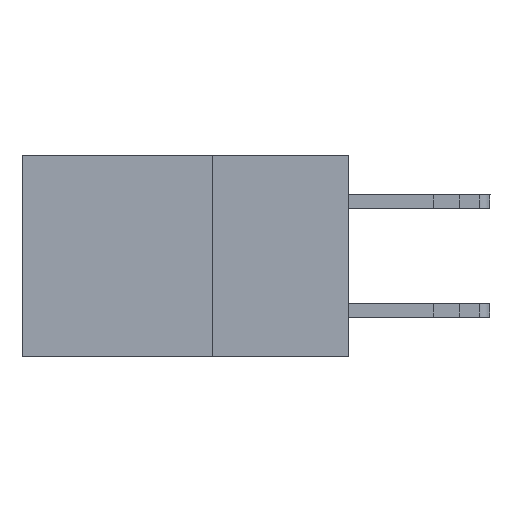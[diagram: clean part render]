
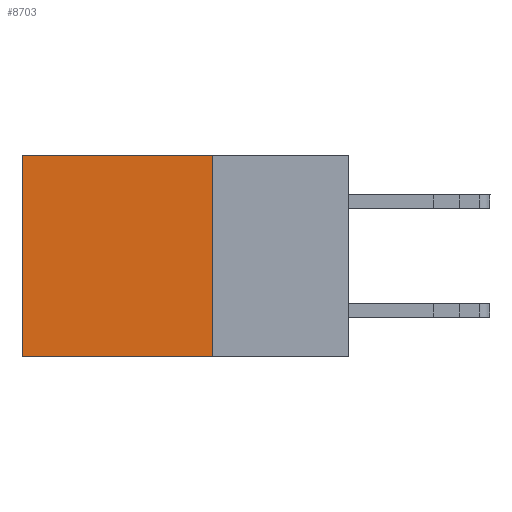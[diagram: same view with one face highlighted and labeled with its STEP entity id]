
A CAD part, left-side view. The second image highlights one B-rep face of the part: STEP entity #8703.
In plain terms, the highlighted planar face has unit normal (-1, 0, 0).
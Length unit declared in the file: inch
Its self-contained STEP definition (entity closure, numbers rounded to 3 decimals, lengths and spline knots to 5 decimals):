
#602 = CARTESIAN_POINT ( 'NONE',  ( 0.298, 0.6, 0. ) ) ;
#836 = EDGE_CURVE ( 'NONE', #10375, #9872, #7836, .T. ) ;
#1963 = DIRECTION ( 'NONE',  ( 0., 0., -1. ) ) ;
#2125 = LINE ( 'NONE', #4439, #6090 ) ;
#2302 = ORIENTED_EDGE ( 'NONE', *, *, #11563, .T. ) ;
#2629 = AXIS2_PLACEMENT_3D ( 'NONE', #14100, #3195, #12896 ) ;
#3061 = LINE ( 'NONE', #7759, #5135 ) ;
#3195 = DIRECTION ( 'NONE',  ( 1., 0., 0. ) ) ;
#3218 = DIRECTION ( 'NONE',  ( 0., 1., 0. ) ) ;
#3538 = CARTESIAN_POINT ( 'NONE',  ( 0.298, 0.25, 0. ) ) ;
#3546 = VECTOR ( 'NONE', #1963, 39.37008 ) ;
#3969 = EDGE_CURVE ( 'NONE', #10375, #10955, #15333, .T. ) ;
#3998 = EDGE_CURVE ( 'NONE', #10955, #11272, #2125, .T. ) ;
#4439 = CARTESIAN_POINT ( 'NONE',  ( 0.298, 0.25, -0.37 ) ) ;
#4466 = ORIENTED_EDGE ( 'NONE', *, *, #3969, .F. ) ;
#5135 = VECTOR ( 'NONE', #8946, 39.37008 ) ;
#6090 = VECTOR ( 'NONE', #9280, 39.37008 ) ;
#7161 = CARTESIAN_POINT ( 'NONE',  ( 0.298, 0.25, 0. ) ) ;
#7759 = CARTESIAN_POINT ( 'NONE',  ( 0.298, 0.6, 0. ) ) ;
#7836 = LINE ( 'NONE', #15156, #8133 ) ;
#8133 = VECTOR ( 'NONE', #3218, 39.37008 ) ;
#8703 = ADVANCED_FACE ( 'NONE', ( #10456 ), #12978, .F. ) ;
#8946 = DIRECTION ( 'NONE',  ( 0., 0., -1. ) ) ;
#9280 = DIRECTION ( 'NONE',  ( 0., 1., 0. ) ) ;
#9506 = ORIENTED_EDGE ( 'NONE', *, *, #836, .T. ) ;
#9872 = VERTEX_POINT ( 'NONE', #602 ) ;
#9889 = EDGE_LOOP ( 'NONE', ( #2302, #13120, #4466, #9506 ) ) ;
#10375 = VERTEX_POINT ( 'NONE', #7161 ) ;
#10456 = FACE_OUTER_BOUND ( 'NONE', #9889, .T. ) ;
#10955 = VERTEX_POINT ( 'NONE', #12223 ) ;
#11272 = VERTEX_POINT ( 'NONE', #14207 ) ;
#11563 = EDGE_CURVE ( 'NONE', #9872, #11272, #3061, .T. ) ;
#12223 = CARTESIAN_POINT ( 'NONE',  ( 0.298, 0.25, -0.37 ) ) ;
#12896 = DIRECTION ( 'NONE',  ( 0., 0., -1. ) ) ;
#12978 = PLANE ( 'NONE',  #2629 ) ;
#13120 = ORIENTED_EDGE ( 'NONE', *, *, #3998, .F. ) ;
#14100 = CARTESIAN_POINT ( 'NONE',  ( 0.298, 0.25, 0. ) ) ;
#14207 = CARTESIAN_POINT ( 'NONE',  ( 0.298, 0.6, -0.37 ) ) ;
#15156 = CARTESIAN_POINT ( 'NONE',  ( 0.298, 0.25, 0. ) ) ;
#15333 = LINE ( 'NONE', #3538, #3546 ) ;
